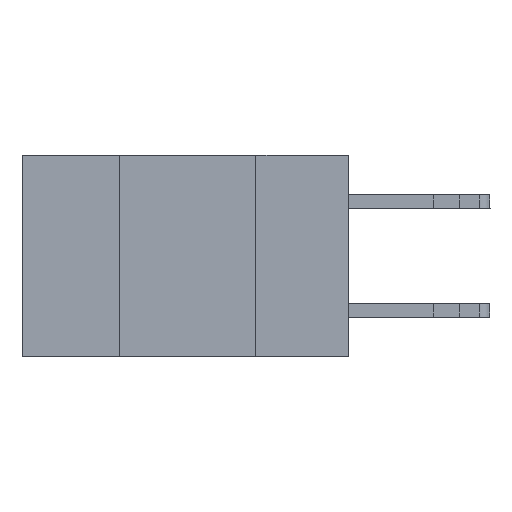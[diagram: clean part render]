
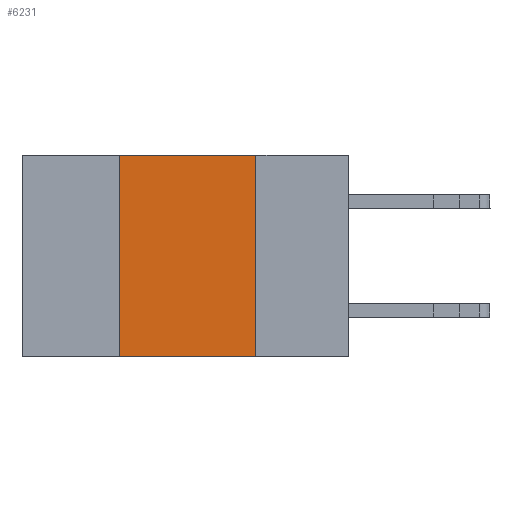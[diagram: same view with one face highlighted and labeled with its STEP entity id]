
A CAD part, left-side view. The second image highlights one B-rep face of the part: STEP entity #6231.
In plain terms, the highlighted planar face has unit normal (-1, 0, 0).
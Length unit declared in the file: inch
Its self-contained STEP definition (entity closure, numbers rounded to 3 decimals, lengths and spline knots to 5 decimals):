
#94 = AXIS2_PLACEMENT_3D ( 'NONE', #11988, #3884, #10387 ) ;
#663 = ORIENTED_EDGE ( 'NONE', *, *, #7944, .F. ) ;
#2051 = LINE ( 'NONE', #17006, #17934 ) ;
#2052 = CARTESIAN_POINT ( 'NONE',  ( 0., 0.42, -0.37 ) ) ;
#3884 = DIRECTION ( 'NONE',  ( 1., 0., 0. ) ) ;
#3957 = CARTESIAN_POINT ( 'NONE',  ( 0., 0.17, -0.37 ) ) ;
#4675 = CARTESIAN_POINT ( 'NONE',  ( 0., 0.17, -0.37 ) ) ;
#4755 = DIRECTION ( 'NONE',  ( 0., -1., 0. ) ) ;
#5508 = ORIENTED_EDGE ( 'NONE', *, *, #19469, .T. ) ;
#5636 = VECTOR ( 'NONE', #8758, 39.37008 ) ;
#6231 = ADVANCED_FACE ( 'NONE', ( #12311 ), #15724, .F. ) ;
#6662 = LINE ( 'NONE', #14779, #10684 ) ;
#7822 = EDGE_LOOP ( 'NONE', ( #12668, #17349, #663, #5508 ) ) ;
#7944 = EDGE_CURVE ( 'NONE', #12689, #8944, #16679, .T. ) ;
#8758 = DIRECTION ( 'NONE',  ( 0., 0., -1. ) ) ;
#8850 = VECTOR ( 'NONE', #18399, 39.37008 ) ;
#8944 = VERTEX_POINT ( 'NONE', #14143 ) ;
#9208 = CARTESIAN_POINT ( 'NONE',  ( 0., 0.42, -0.37 ) ) ;
#10387 = DIRECTION ( 'NONE',  ( 0., 0., -1. ) ) ;
#10684 = VECTOR ( 'NONE', #4755, 39.37008 ) ;
#11644 = EDGE_CURVE ( 'NONE', #8944, #15679, #2051, .T. ) ;
#11988 = CARTESIAN_POINT ( 'NONE',  ( 0., 0.6, 0. ) ) ;
#12001 = CARTESIAN_POINT ( 'NONE',  ( 0., 0.17, 0. ) ) ;
#12311 = FACE_OUTER_BOUND ( 'NONE', #7822, .T. ) ;
#12668 = ORIENTED_EDGE ( 'NONE', *, *, #13359, .F. ) ;
#12689 = VERTEX_POINT ( 'NONE', #9208 ) ;
#13359 = EDGE_CURVE ( 'NONE', #15679, #18958, #14949, .T. ) ;
#13366 = DIRECTION ( 'NONE',  ( 0., -1., 0. ) ) ;
#14143 = CARTESIAN_POINT ( 'NONE',  ( 0., 0.42, 0. ) ) ;
#14779 = CARTESIAN_POINT ( 'NONE',  ( 0., 0.6, -0.37 ) ) ;
#14949 = LINE ( 'NONE', #3957, #5636 ) ;
#15679 = VERTEX_POINT ( 'NONE', #12001 ) ;
#15724 = PLANE ( 'NONE',  #94 ) ;
#16679 = LINE ( 'NONE', #2052, #8850 ) ;
#17006 = CARTESIAN_POINT ( 'NONE',  ( 0., 0.6, 0. ) ) ;
#17349 = ORIENTED_EDGE ( 'NONE', *, *, #11644, .F. ) ;
#17934 = VECTOR ( 'NONE', #13366, 39.37008 ) ;
#18399 = DIRECTION ( 'NONE',  ( 0., 0., 1. ) ) ;
#18958 = VERTEX_POINT ( 'NONE', #4675 ) ;
#19469 = EDGE_CURVE ( 'NONE', #12689, #18958, #6662, .T. ) ;
